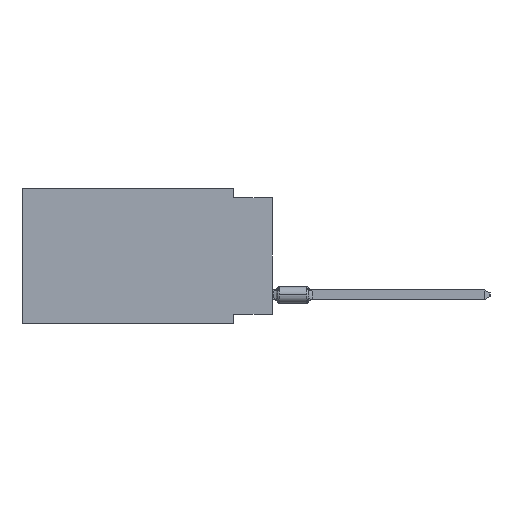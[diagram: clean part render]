
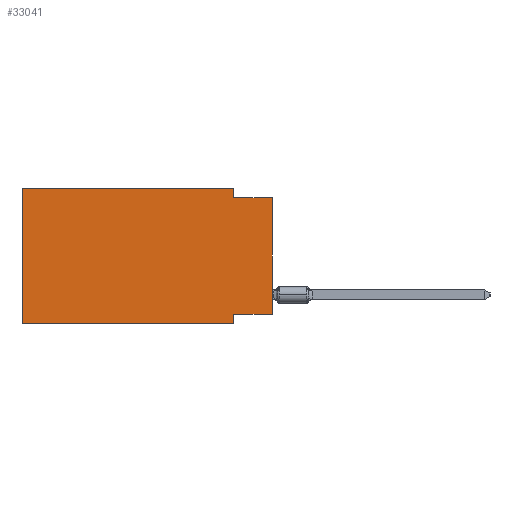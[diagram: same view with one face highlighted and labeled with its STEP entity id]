
A CAD part, left-side view. The second image highlights one B-rep face of the part: STEP entity #33041.
In plain terms, the highlighted planar face has unit normal (-1, 0, 0).
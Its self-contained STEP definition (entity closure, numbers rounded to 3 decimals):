
#182 = ORIENTED_EDGE ( 'NONE', *, *, #15249, .T. ) ;
#323 = CARTESIAN_POINT ( 'NONE',  ( 0., 2.54, -8.255 ) ) ;
#394 = VECTOR ( 'NONE', #41037, 1000. ) ;
#1631 = VERTEX_POINT ( 'NONE', #14768 ) ;
#2678 = ORIENTED_EDGE ( 'NONE', *, *, #26780, .F. ) ;
#5042 = VERTEX_POINT ( 'NONE', #14355 ) ;
#5315 = DIRECTION ( 'NONE',  ( 0., -1., 0. ) ) ;
#7307 = VECTOR ( 'NONE', #36044, 1000. ) ;
#9434 = DIRECTION ( 'NONE',  ( 0., 0., -1. ) ) ;
#9679 = VERTEX_POINT ( 'NONE', #13213 ) ;
#9781 = EDGE_CURVE ( 'NONE', #41899, #20503, #20176, .T. ) ;
#10306 = LINE ( 'NONE', #24018, #11623 ) ;
#10704 = CARTESIAN_POINT ( 'NONE',  ( 0., 16.383, 0. ) ) ;
#11623 = VECTOR ( 'NONE', #20639, 1000. ) ;
#13213 = CARTESIAN_POINT ( 'NONE',  ( 0., 2.54, 0. ) ) ;
#14096 = VERTEX_POINT ( 'NONE', #19354 ) ;
#14355 = CARTESIAN_POINT ( 'NONE',  ( 0., 2.54, -0.635 ) ) ;
#14768 = CARTESIAN_POINT ( 'NONE',  ( 0., 16.383, 0. ) ) ;
#15249 = EDGE_CURVE ( 'NONE', #28029, #21072, #22889, .T. ) ;
#15422 = LINE ( 'NONE', #35859, #43353 ) ;
#19080 = DIRECTION ( 'NONE',  ( 0., -1., 0. ) ) ;
#19354 = CARTESIAN_POINT ( 'NONE',  ( 0., 0., -0.635 ) ) ;
#19861 = CARTESIAN_POINT ( 'NONE',  ( 0., 2.54, -8.89 ) ) ;
#19980 = DIRECTION ( 'NONE',  ( 1., 0., 0. ) ) ;
#20176 = LINE ( 'NONE', #36370, #22978 ) ;
#20503 = VERTEX_POINT ( 'NONE', #323 ) ;
#20639 = DIRECTION ( 'NONE',  ( 0., 0., 1. ) ) ;
#20862 = VECTOR ( 'NONE', #19080, 1000. ) ;
#21015 = VECTOR ( 'NONE', #29667, 1000. ) ;
#21072 = VERTEX_POINT ( 'NONE', #19861 ) ;
#22279 = AXIS2_PLACEMENT_3D ( 'NONE', #40867, #19980, #9434 ) ;
#22676 = DIRECTION ( 'NONE',  ( 0., 1., 0. ) ) ;
#22889 = LINE ( 'NONE', #36574, #20862 ) ;
#22895 = ORIENTED_EDGE ( 'NONE', *, *, #35487, .F. ) ;
#22978 = VECTOR ( 'NONE', #22676, 1000. ) ;
#23427 = CARTESIAN_POINT ( 'NONE',  ( 0., 0., -8.255 ) ) ;
#23501 = ORIENTED_EDGE ( 'NONE', *, *, #30851, .F. ) ;
#23735 = ORIENTED_EDGE ( 'NONE', *, *, #37386, .F. ) ;
#23743 = LINE ( 'NONE', #10704, #394 ) ;
#24018 = CARTESIAN_POINT ( 'NONE',  ( 0., 0., 0. ) ) ;
#26508 = PLANE ( 'NONE',  #22279 ) ;
#26735 = LINE ( 'NONE', #40872, #21015 ) ;
#26780 = EDGE_CURVE ( 'NONE', #5042, #14096, #40086, .T. ) ;
#28029 = VERTEX_POINT ( 'NONE', #44389 ) ;
#28668 = EDGE_LOOP ( 'NONE', ( #30997, #2678, #23501, #23735, #34814, #182, #22895, #38373 ) ) ;
#29667 = DIRECTION ( 'NONE',  ( 0., 0., -1. ) ) ;
#29980 = LINE ( 'NONE', #40090, #32575 ) ;
#30851 = EDGE_CURVE ( 'NONE', #9679, #5042, #29980, .T. ) ;
#30997 = ORIENTED_EDGE ( 'NONE', *, *, #39445, .T. ) ;
#31840 = EDGE_CURVE ( 'NONE', #28029, #1631, #23743, .T. ) ;
#32575 = VECTOR ( 'NONE', #36047, 1000. ) ;
#32905 = CARTESIAN_POINT ( 'NONE',  ( 0., 0., -0.635 ) ) ;
#33041 = ADVANCED_FACE ( 'NONE', ( #40206 ), #26508, .F. ) ;
#34814 = ORIENTED_EDGE ( 'NONE', *, *, #31840, .F. ) ;
#35487 = EDGE_CURVE ( 'NONE', #20503, #21072, #26735, .T. ) ;
#35859 = CARTESIAN_POINT ( 'NONE',  ( 0., 16.383, 0. ) ) ;
#36044 = DIRECTION ( 'NONE',  ( 0., -1., 0. ) ) ;
#36047 = DIRECTION ( 'NONE',  ( 0., 0., -1. ) ) ;
#36370 = CARTESIAN_POINT ( 'NONE',  ( 0., 0., -8.255 ) ) ;
#36574 = CARTESIAN_POINT ( 'NONE',  ( 0., 16.383, -8.89 ) ) ;
#37386 = EDGE_CURVE ( 'NONE', #1631, #9679, #15422, .T. ) ;
#38373 = ORIENTED_EDGE ( 'NONE', *, *, #9781, .F. ) ;
#39445 = EDGE_CURVE ( 'NONE', #41899, #14096, #10306, .T. ) ;
#40086 = LINE ( 'NONE', #32905, #7307 ) ;
#40090 = CARTESIAN_POINT ( 'NONE',  ( 0., 2.54, 0. ) ) ;
#40206 = FACE_OUTER_BOUND ( 'NONE', #28668, .T. ) ;
#40867 = CARTESIAN_POINT ( 'NONE',  ( 0., 16.383, 0. ) ) ;
#40872 = CARTESIAN_POINT ( 'NONE',  ( 0., 2.54, -8.89 ) ) ;
#41037 = DIRECTION ( 'NONE',  ( 0., 0., 1. ) ) ;
#41899 = VERTEX_POINT ( 'NONE', #23427 ) ;
#43353 = VECTOR ( 'NONE', #5315, 1000. ) ;
#44389 = CARTESIAN_POINT ( 'NONE',  ( 0., 16.383, -8.89 ) ) ;
